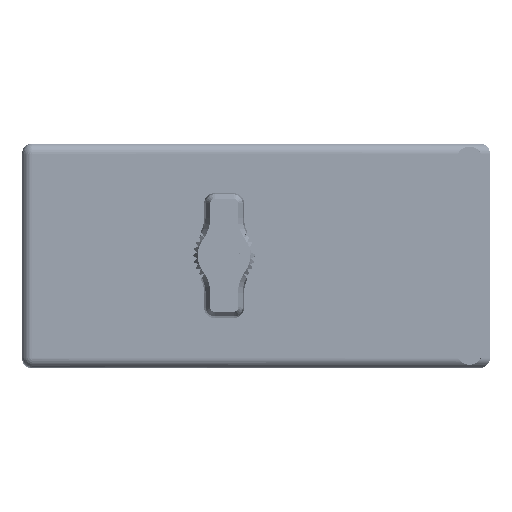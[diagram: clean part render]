
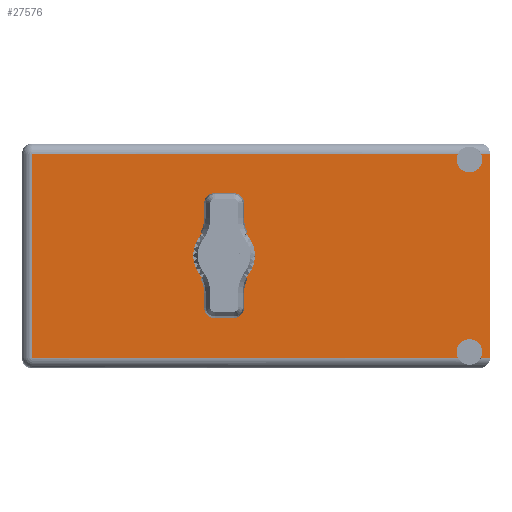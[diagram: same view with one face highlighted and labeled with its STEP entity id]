
A CAD part, top view. The second image highlights one B-rep face of the part: STEP entity #27576.
In plain terms, the highlighted face is planar.
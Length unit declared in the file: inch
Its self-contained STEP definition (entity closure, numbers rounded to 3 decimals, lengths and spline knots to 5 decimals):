
#318 = CARTESIAN_POINT ( 'NONE',  ( 3.12833, 2.03, -0.07 ) ) ;
#2351 = ORIENTED_EDGE ( 'NONE', *, *, #80366, .F. ) ;
#2606 = DIRECTION ( 'NONE',  ( 0., 1., 0. ) ) ;
#3024 = EDGE_CURVE ( 'NONE', #20303, #42498, #43313, .T. ) ;
#3725 = EDGE_CURVE ( 'NONE', #67994, #5532, #72967, .T. ) ;
#5532 = VERTEX_POINT ( 'NONE', #38286 ) ;
#8621 = EDGE_CURVE ( 'NONE', #59083, #20303, #66941, .T. ) ;
#9962 = ORIENTED_EDGE ( 'NONE', *, *, #77700, .F. ) ;
#10232 = VERTEX_POINT ( 'NONE', #14737 ) ;
#10554 = DIRECTION ( 'NONE',  ( 0., 1., 0. ) ) ;
#10634 = CARTESIAN_POINT ( 'NONE',  ( 3.19, 2.03, -0.07 ) ) ;
#10709 = CARTESIAN_POINT ( 'NONE',  ( 1.3775, 2.03, -0.595 ) ) ;
#11428 = CIRCLE ( 'NONE', #89782, 0.17 ) ;
#11450 = CARTESIAN_POINT ( 'NONE',  ( 3.05, 2.03, -0.109 ) ) ;
#13669 = DIRECTION ( 'NONE',  ( 0., 0., 1. ) ) ;
#14737 = CARTESIAN_POINT ( 'NONE',  ( 1.3775, 2.03, -0.935 ) ) ;
#16571 = VERTEX_POINT ( 'NONE', #10634 ) ;
#16851 = DIRECTION ( 'NONE',  ( 0., 0., 1. ) ) ;
#16868 = CARTESIAN_POINT ( 'NONE',  ( 2.97167, 2.03, -0.07 ) ) ;
#18647 = EDGE_CURVE ( 'NONE', #104891, #16571, #108148, .T. ) ;
#19230 = AXIS2_PLACEMENT_3D ( 'NONE', #79244, #10554, #52729 ) ;
#19819 = EDGE_LOOP ( 'NONE', ( #82035, #61123, #52873, #35310, #2351, #95108, #46443, #9962, #43145, #36138 ) ) ;
#20303 = VERTEX_POINT ( 'NONE', #98213 ) ;
#20343 = VECTOR ( 'NONE', #52259, 39.37008 ) ;
#21124 = LINE ( 'NONE', #63214, #25003 ) ;
#23667 = CIRCLE ( 'NONE', #33299, 0.0875 ) ;
#25003 = VECTOR ( 'NONE', #54762, 39.37008 ) ;
#25207 = CARTESIAN_POINT ( 'NONE',  ( 0., 2.03, -1.46 ) ) ;
#27576 = ADVANCED_FACE ( 'NONE', ( #64989, #29258 ), #97192, .T. ) ;
#28285 = AXIS2_PLACEMENT_3D ( 'NONE', #58968, #33824, #100729 ) ;
#28698 = VECTOR ( 'NONE', #50319, 39.37008 ) ;
#29258 = FACE_OUTER_BOUND ( 'NONE', #19819, .T. ) ;
#30875 = EDGE_CURVE ( 'NONE', #88696, #5532, #40488, .T. ) ;
#32914 = EDGE_CURVE ( 'NONE', #60155, #10232, #83771, .T. ) ;
#33299 = AXIS2_PLACEMENT_3D ( 'NONE', #11450, #2606, #37332 ) ;
#33824 = DIRECTION ( 'NONE',  ( 0., 1., 0. ) ) ;
#35310 = ORIENTED_EDGE ( 'NONE', *, *, #18647, .T. ) ;
#36138 = ORIENTED_EDGE ( 'NONE', *, *, #8621, .T. ) ;
#37332 = DIRECTION ( 'NONE',  ( 0., 0., 1. ) ) ;
#38286 = CARTESIAN_POINT ( 'NONE',  ( 3.12833, 2.03, -1.46 ) ) ;
#38766 = CARTESIAN_POINT ( 'NONE',  ( 0.07, 2.03, -1.53 ) ) ;
#40229 = CARTESIAN_POINT ( 'NONE',  ( 3.19, 2.03, -1.46 ) ) ;
#40488 = CIRCLE ( 'NONE', #28285, 0.0875 ) ;
#42126 = AXIS2_PLACEMENT_3D ( 'NONE', #63624, #64341, #64697 ) ;
#42498 = VERTEX_POINT ( 'NONE', #16868 ) ;
#43145 = ORIENTED_EDGE ( 'NONE', *, *, #103274, .T. ) ;
#43144 = DIRECTION ( 'NONE',  ( 0., 0., 1. ) ) ;
#43172 = CARTESIAN_POINT ( 'NONE',  ( 1.3775, 2.03, -0.765 ) ) ;
#43313 = LINE ( 'NONE', #100203, #28698 ) ;
#44083 = EDGE_CURVE ( 'NONE', #56441, #42498, #23667, .T. ) ;
#45337 = CARTESIAN_POINT ( 'NONE',  ( 3.05, 2.03, -1.3335 ) ) ;
#45825 = CARTESIAN_POINT ( 'NONE',  ( 2.97167, 2.03, -1.46 ) ) ;
#46443 = ORIENTED_EDGE ( 'NONE', *, *, #30875, .F. ) ;
#48110 = ORIENTED_EDGE ( 'NONE', *, *, #32914, .F. ) ;
#50319 = DIRECTION ( 'NONE',  ( 1., 0., 0. ) ) ;
#51020 = CARTESIAN_POINT ( 'NONE',  ( 3.05, 2.03, -0.1965 ) ) ;
#52139 = CIRCLE ( 'NONE', #42126, 0.0875 ) ;
#52259 = DIRECTION ( 'NONE',  ( -1., 0., 0. ) ) ;
#52729 = DIRECTION ( 'NONE',  ( 0., 0., 1. ) ) ;
#52873 = ORIENTED_EDGE ( 'NONE', *, *, #65658, .F. ) ;
#54762 = DIRECTION ( 'NONE',  ( 0., 0., 1. ) ) ;
#56441 = VERTEX_POINT ( 'NONE', #51020 ) ;
#58968 = CARTESIAN_POINT ( 'NONE',  ( 3.05, 2.03, -1.421 ) ) ;
#58992 = EDGE_CURVE ( 'NONE', #10232, #60155, #11428, .T. ) ;
#59083 = VERTEX_POINT ( 'NONE', #59372 ) ;
#59372 = CARTESIAN_POINT ( 'NONE',  ( 0.07, 2.03, -1.46 ) ) ;
#60103 = DIRECTION ( 'NONE',  ( 0., 1., 0. ) ) ;
#60155 = VERTEX_POINT ( 'NONE', #10709 ) ;
#61123 = ORIENTED_EDGE ( 'NONE', *, *, #44083, .F. ) ;
#61567 = CARTESIAN_POINT ( 'NONE',  ( 3.05, 2.03, -0.109 ) ) ;
#63214 = CARTESIAN_POINT ( 'NONE',  ( 3.19, 2.03, 0. ) ) ;
#63310 = DIRECTION ( 'NONE',  ( 1., 0., 0. ) ) ;
#63624 = CARTESIAN_POINT ( 'NONE',  ( 3.05, 2.03, -1.421 ) ) ;
#64208 = DIRECTION ( 'NONE',  ( 0., 0., 1. ) ) ;
#64341 = DIRECTION ( 'NONE',  ( 0., 1., 0. ) ) ;
#64697 = DIRECTION ( 'NONE',  ( 0., 0., 1. ) ) ;
#64833 = ORIENTED_EDGE ( 'NONE', *, *, #58992, .F. ) ;
#64989 = FACE_BOUND ( 'NONE', #90189, .T. ) ;
#65658 = EDGE_CURVE ( 'NONE', #104891, #56441, #86444, .T. ) ;
#66941 = LINE ( 'NONE', #38766, #109244 ) ;
#67994 = VERTEX_POINT ( 'NONE', #40229 ) ;
#68491 = DIRECTION ( 'NONE',  ( -1., 0., 0. ) ) ;
#70561 = LINE ( 'NONE', #104311, #20343 ) ;
#72967 = LINE ( 'NONE', #25207, #100800 ) ;
#77700 = EDGE_CURVE ( 'NONE', #90230, #88696, #52139, .T. ) ;
#79244 = CARTESIAN_POINT ( 'NONE',  ( 1.3775, 2.03, -0.765 ) ) ;
#80366 = EDGE_CURVE ( 'NONE', #67994, #16571, #21124, .T. ) ;
#82035 = ORIENTED_EDGE ( 'NONE', *, *, #3024, .T. ) ;
#83771 = CIRCLE ( 'NONE', #19230, 0.17 ) ;
#85629 = VECTOR ( 'NONE', #63310, 39.37008 ) ;
#86444 = CIRCLE ( 'NONE', #91737, 0.0875 ) ;
#88322 = DIRECTION ( 'NONE',  ( 0., 1., 0. ) ) ;
#88420 = CARTESIAN_POINT ( 'NONE',  ( 3.19, 2.03, -0.07 ) ) ;
#88696 = VERTEX_POINT ( 'NONE', #45337 ) ;
#89782 = AXIS2_PLACEMENT_3D ( 'NONE', #43172, #101869, #16851 ) ;
#90189 = EDGE_LOOP ( 'NONE', ( #48110, #64833 ) ) ;
#90230 = VERTEX_POINT ( 'NONE', #45825 ) ;
#91737 = AXIS2_PLACEMENT_3D ( 'NONE', #61567, #60103, #43144 ) ;
#95108 = ORIENTED_EDGE ( 'NONE', *, *, #3725, .T. ) ;
#97192 = PLANE ( 'NONE',  #108110 ) ;
#98213 = CARTESIAN_POINT ( 'NONE',  ( 0.07, 2.03, -0.07 ) ) ;
#98280 = CARTESIAN_POINT ( 'NONE',  ( 0., 2.03, -1.53 ) ) ;
#100203 = CARTESIAN_POINT ( 'NONE',  ( 3.19, 2.03, -0.07 ) ) ;
#100729 = DIRECTION ( 'NONE',  ( 0., 0., 1. ) ) ;
#100800 = VECTOR ( 'NONE', #68491, 39.37008 ) ;
#101869 = DIRECTION ( 'NONE',  ( 0., 1., 0. ) ) ;
#103274 = EDGE_CURVE ( 'NONE', #90230, #59083, #70561, .T. ) ;
#104311 = CARTESIAN_POINT ( 'NONE',  ( 0., 2.03, -1.46 ) ) ;
#104891 = VERTEX_POINT ( 'NONE', #318 ) ;
#108110 = AXIS2_PLACEMENT_3D ( 'NONE', #98280, #88322, #13669 ) ;
#108148 = LINE ( 'NONE', #88420, #85629 ) ;
#109244 = VECTOR ( 'NONE', #64208, 39.37008 ) ;
